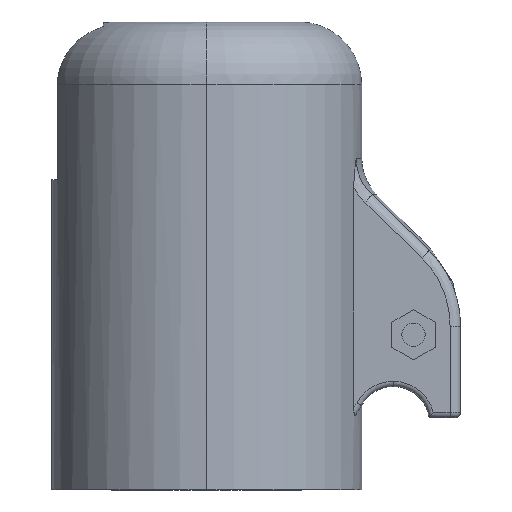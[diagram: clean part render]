
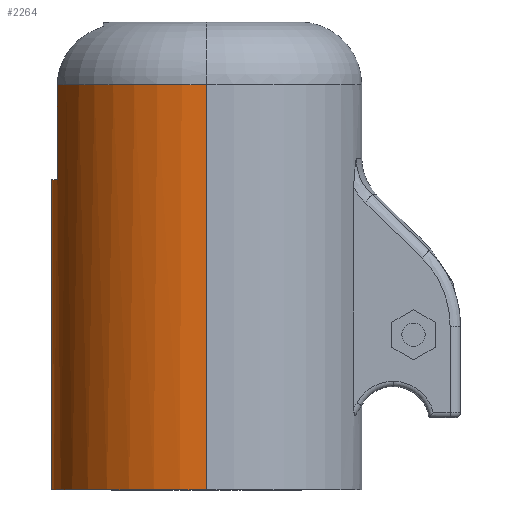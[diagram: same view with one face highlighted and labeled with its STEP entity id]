
A CAD part, left-side view. The second image highlights one B-rep face of the part: STEP entity #2264.
In plain terms, the highlighted cylindrical face has radius 15 mm (diameter 30 mm), a partial arc.
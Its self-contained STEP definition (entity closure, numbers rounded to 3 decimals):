
#33 = DIRECTION ( 'NONE',  ( 0., 0., -1. ) ) ;
#182 = LINE ( 'NONE', #7252, #7603 ) ;
#240 = DIRECTION ( 'NONE',  ( 0., 0., -1. ) ) ;
#361 = ORIENTED_EDGE ( 'NONE', *, *, #5931, .T. ) ;
#512 = CARTESIAN_POINT ( 'NONE',  ( 0., 0., 40. ) ) ;
#529 = CIRCLE ( 'NONE', #6940, 15. ) ;
#631 = CARTESIAN_POINT ( 'NONE',  ( 15., 0., 39.176 ) ) ;
#674 = CARTESIAN_POINT ( 'NONE',  ( -4.115, 14.424, 39.176 ) ) ;
#922 = VERTEX_POINT ( 'NONE', #2383 ) ;
#988 = VECTOR ( 'NONE', #33, 1000. ) ;
#1030 = DIRECTION ( 'NONE',  ( 0., 0., 1. ) ) ;
#1305 = ORIENTED_EDGE ( 'NONE', *, *, #4435, .T. ) ;
#1566 = VERTEX_POINT ( 'NONE', #6616 ) ;
#1821 = VECTOR ( 'NONE', #7191, 1000. ) ;
#1829 = VECTOR ( 'NONE', #3829, 1000. ) ;
#1919 = ORIENTED_EDGE ( 'NONE', *, *, #6644, .T. ) ;
#2102 = DIRECTION ( 'NONE',  ( 0., 0., -1. ) ) ;
#2264 = ADVANCED_FACE ( 'NONE', ( #7343 ), #5616, .T. ) ;
#2278 = VERTEX_POINT ( 'NONE', #2834 ) ;
#2287 = ORIENTED_EDGE ( 'NONE', *, *, #6505, .T. ) ;
#2383 = CARTESIAN_POINT ( 'NONE',  ( -4.115, 14.424, 30. ) ) ;
#2440 = AXIS2_PLACEMENT_3D ( 'NONE', #512, #5748, #7525 ) ;
#2452 = DIRECTION ( 'NONE',  ( 0., 0., 1. ) ) ;
#2529 = AXIS2_PLACEMENT_3D ( 'NONE', #4553, #1030, #5144 ) ;
#2662 = ORIENTED_EDGE ( 'NONE', *, *, #6358, .F. ) ;
#2834 = CARTESIAN_POINT ( 'NONE',  ( 4.115, 14.424, 30. ) ) ;
#3161 = CIRCLE ( 'NONE', #3382, 15. ) ;
#3235 = CARTESIAN_POINT ( 'NONE',  ( 4.115, 14.424, 30. ) ) ;
#3279 = CARTESIAN_POINT ( 'NONE',  ( 15., 0., 0. ) ) ;
#3360 = LINE ( 'NONE', #3235, #1829 ) ;
#3382 = AXIS2_PLACEMENT_3D ( 'NONE', #6920, #3388, #7508 ) ;
#3388 = DIRECTION ( 'NONE',  ( 0., 0., -1. ) ) ;
#3414 = ORIENTED_EDGE ( 'NONE', *, *, #4278, .T. ) ;
#3711 = LINE ( 'NONE', #4849, #1821 ) ;
#3829 = DIRECTION ( 'NONE',  ( 0., 0., 1. ) ) ;
#3892 = AXIS2_PLACEMENT_3D ( 'NONE', #6007, #2452, #6585 ) ;
#4060 = VERTEX_POINT ( 'NONE', #6151 ) ;
#4239 = ORIENTED_EDGE ( 'NONE', *, *, #4846, .F. ) ;
#4278 = EDGE_CURVE ( 'NONE', #2278, #1566, #3360, .T. ) ;
#4435 = EDGE_CURVE ( 'NONE', #1566, #6598, #3161, .T. ) ;
#4553 = CARTESIAN_POINT ( 'NONE',  ( 0., 0., 30. ) ) ;
#4597 = VERTEX_POINT ( 'NONE', #674 ) ;
#4846 = EDGE_CURVE ( 'NONE', #2278, #922, #4860, .T. ) ;
#4849 = CARTESIAN_POINT ( 'NONE',  ( -4.115, 14.424, 30. ) ) ;
#4860 = CIRCLE ( 'NONE', #2529, 15. ) ;
#4867 = CIRCLE ( 'NONE', #3892, 15. ) ;
#4898 = VERTEX_POINT ( 'NONE', #5212 ) ;
#5144 = DIRECTION ( 'NONE',  ( 1., 0., 0. ) ) ;
#5212 = CARTESIAN_POINT ( 'NONE',  ( -15., 0., 0. ) ) ;
#5388 = EDGE_CURVE ( 'NONE', #922, #4597, #3711, .T. ) ;
#5479 = LINE ( 'NONE', #7061, #988 ) ;
#5616 = CYLINDRICAL_SURFACE ( 'NONE', #2440, 15. ) ;
#5646 = CARTESIAN_POINT ( 'NONE',  ( 0., 0., 39.176 ) ) ;
#5748 = DIRECTION ( 'NONE',  ( 0., 0., -1. ) ) ;
#5931 = EDGE_CURVE ( 'NONE', #4060, #4597, #529, .T. ) ;
#5970 = VERTEX_POINT ( 'NONE', #3279 ) ;
#6007 = CARTESIAN_POINT ( 'NONE',  ( 0., 0., 0. ) ) ;
#6151 = CARTESIAN_POINT ( 'NONE',  ( -15., 0., 39.176 ) ) ;
#6230 = DIRECTION ( 'NONE',  ( 1., 0., 0. ) ) ;
#6358 = EDGE_CURVE ( 'NONE', #4060, #4898, #5479, .T. ) ;
#6505 = EDGE_CURVE ( 'NONE', #5970, #4898, #4867, .T. ) ;
#6585 = DIRECTION ( 'NONE',  ( 1., 0., 0. ) ) ;
#6598 = VERTEX_POINT ( 'NONE', #631 ) ;
#6616 = CARTESIAN_POINT ( 'NONE',  ( 4.115, 14.424, 39.176 ) ) ;
#6644 = EDGE_CURVE ( 'NONE', #6598, #5970, #182, .T. ) ;
#6710 = EDGE_LOOP ( 'NONE', ( #1305, #1919, #2287, #2662, #361, #6793, #4239, #3414 ) ) ;
#6793 = ORIENTED_EDGE ( 'NONE', *, *, #5388, .F. ) ;
#6920 = CARTESIAN_POINT ( 'NONE',  ( 0., 0., 39.176 ) ) ;
#6940 = AXIS2_PLACEMENT_3D ( 'NONE', #5646, #2102, #6230 ) ;
#7061 = CARTESIAN_POINT ( 'NONE',  ( -15., 0., 40. ) ) ;
#7191 = DIRECTION ( 'NONE',  ( 0., 0., 1. ) ) ;
#7252 = CARTESIAN_POINT ( 'NONE',  ( 15., 0., 40. ) ) ;
#7343 = FACE_OUTER_BOUND ( 'NONE', #6710, .T. ) ;
#7508 = DIRECTION ( 'NONE',  ( 1., 0., 0. ) ) ;
#7525 = DIRECTION ( 'NONE',  ( -1., 0., 0. ) ) ;
#7603 = VECTOR ( 'NONE', #240, 1000. ) ;
